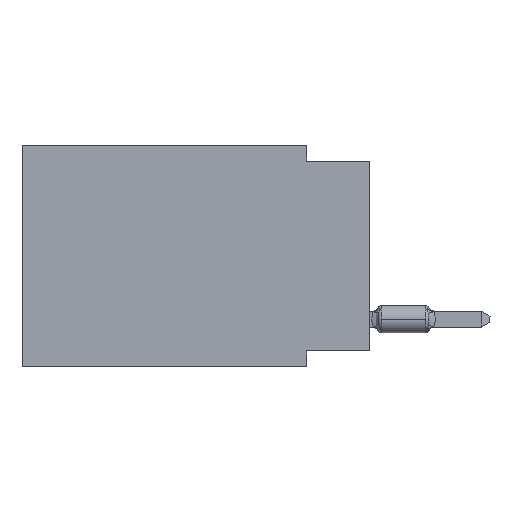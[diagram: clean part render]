
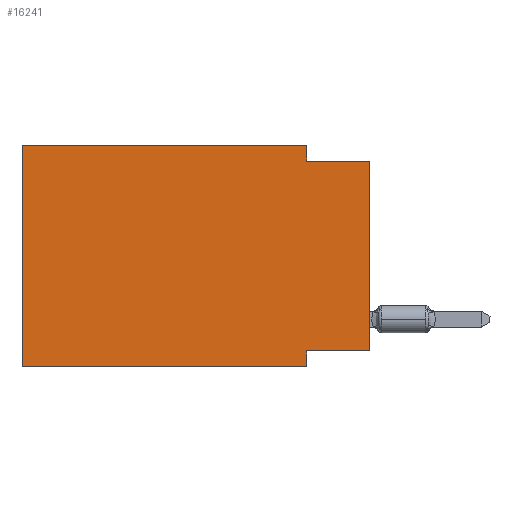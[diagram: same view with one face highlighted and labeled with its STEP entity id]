
A CAD part, left-side view. The second image highlights one B-rep face of the part: STEP entity #16241.
In plain terms, the highlighted planar face has unit normal (-1, 0, 0).
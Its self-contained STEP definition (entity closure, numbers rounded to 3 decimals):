
#185 = CARTESIAN_POINT ( 'NONE',  ( 0., 2.54, 0. ) ) ;
#246 = DIRECTION ( 'NONE',  ( 1., 0., 0. ) ) ;
#459 = CARTESIAN_POINT ( 'NONE',  ( 0., 0., -8.255 ) ) ;
#658 = LINE ( 'NONE', #14765, #14138 ) ;
#840 = VERTEX_POINT ( 'NONE', #3862 ) ;
#853 = VECTOR ( 'NONE', #5215, 1000. ) ;
#1459 = LINE ( 'NONE', #459, #10070 ) ;
#1527 = ORIENTED_EDGE ( 'NONE', *, *, #9915, .F. ) ;
#1926 = LINE ( 'NONE', #8041, #5080 ) ;
#2271 = LINE ( 'NONE', #2593, #2437 ) ;
#2437 = VECTOR ( 'NONE', #10041, 1000. ) ;
#2534 = EDGE_CURVE ( 'NONE', #9125, #10324, #11504, .T. ) ;
#2593 = CARTESIAN_POINT ( 'NONE',  ( 0., 2.54, -8.89 ) ) ;
#2864 = VERTEX_POINT ( 'NONE', #6585 ) ;
#2970 = ORIENTED_EDGE ( 'NONE', *, *, #7708, .F. ) ;
#3040 = VERTEX_POINT ( 'NONE', #4750 ) ;
#3373 = DIRECTION ( 'NONE',  ( 0., -1., 0. ) ) ;
#3577 = ORIENTED_EDGE ( 'NONE', *, *, #12218, .F. ) ;
#3752 = VECTOR ( 'NONE', #6814, 1000. ) ;
#3862 = CARTESIAN_POINT ( 'NONE',  ( 0., 13.97, -8.89 ) ) ;
#3876 = EDGE_LOOP ( 'NONE', ( #8422, #14463, #13564, #1527, #2970, #4227, #12075, #3577 ) ) ;
#4227 = ORIENTED_EDGE ( 'NONE', *, *, #6382, .T. ) ;
#4547 = CARTESIAN_POINT ( 'NONE',  ( 0., 2.54, -0.635 ) ) ;
#4742 = CARTESIAN_POINT ( 'NONE',  ( 0., 13.97, 0. ) ) ;
#4750 = CARTESIAN_POINT ( 'NONE',  ( 0., 2.54, -8.89 ) ) ;
#5080 = VECTOR ( 'NONE', #10938, 1000. ) ;
#5215 = DIRECTION ( 'NONE',  ( 0., 0., -1. ) ) ;
#5586 = VECTOR ( 'NONE', #8556, 1000. ) ;
#5631 = EDGE_CURVE ( 'NONE', #10324, #10305, #658, .T. ) ;
#6362 = DIRECTION ( 'NONE',  ( 0., 0., -1. ) ) ;
#6382 = EDGE_CURVE ( 'NONE', #840, #3040, #8968, .T. ) ;
#6585 = CARTESIAN_POINT ( 'NONE',  ( 0., 13.97, 0. ) ) ;
#6814 = DIRECTION ( 'NONE',  ( 0., 0., 1. ) ) ;
#7611 = VERTEX_POINT ( 'NONE', #14409 ) ;
#7708 = EDGE_CURVE ( 'NONE', #840, #2864, #16056, .T. ) ;
#8041 = CARTESIAN_POINT ( 'NONE',  ( 0., 13.97, 0. ) ) ;
#8422 = ORIENTED_EDGE ( 'NONE', *, *, #12714, .T. ) ;
#8556 = DIRECTION ( 'NONE',  ( 0., 0., 1. ) ) ;
#8935 = PLANE ( 'NONE',  #9315 ) ;
#8968 = LINE ( 'NONE', #15800, #10439 ) ;
#9125 = VERTEX_POINT ( 'NONE', #13109 ) ;
#9308 = LINE ( 'NONE', #10715, #3752 ) ;
#9315 = AXIS2_PLACEMENT_3D ( 'NONE', #12565, #246, #6362 ) ;
#9582 = VERTEX_POINT ( 'NONE', #15802 ) ;
#9612 = EDGE_CURVE ( 'NONE', #7611, #3040, #2271, .T. ) ;
#9915 = EDGE_CURVE ( 'NONE', #2864, #9125, #1926, .T. ) ;
#10041 = DIRECTION ( 'NONE',  ( 0., 0., -1. ) ) ;
#10070 = VECTOR ( 'NONE', #11957, 1000. ) ;
#10305 = VERTEX_POINT ( 'NONE', #15850 ) ;
#10324 = VERTEX_POINT ( 'NONE', #4547 ) ;
#10439 = VECTOR ( 'NONE', #10864, 1000. ) ;
#10715 = CARTESIAN_POINT ( 'NONE',  ( 0., 0., 0. ) ) ;
#10864 = DIRECTION ( 'NONE',  ( 0., -1., 0. ) ) ;
#10938 = DIRECTION ( 'NONE',  ( 0., -1., 0. ) ) ;
#11504 = LINE ( 'NONE', #185, #853 ) ;
#11957 = DIRECTION ( 'NONE',  ( 0., 1., 0. ) ) ;
#12075 = ORIENTED_EDGE ( 'NONE', *, *, #9612, .F. ) ;
#12218 = EDGE_CURVE ( 'NONE', #9582, #7611, #1459, .T. ) ;
#12565 = CARTESIAN_POINT ( 'NONE',  ( 0., 13.97, 0. ) ) ;
#12714 = EDGE_CURVE ( 'NONE', #9582, #10305, #9308, .T. ) ;
#13109 = CARTESIAN_POINT ( 'NONE',  ( 0., 2.54, 0. ) ) ;
#13564 = ORIENTED_EDGE ( 'NONE', *, *, #2534, .F. ) ;
#13710 = FACE_OUTER_BOUND ( 'NONE', #3876, .T. ) ;
#14138 = VECTOR ( 'NONE', #3373, 1000. ) ;
#14409 = CARTESIAN_POINT ( 'NONE',  ( 0., 2.54, -8.255 ) ) ;
#14463 = ORIENTED_EDGE ( 'NONE', *, *, #5631, .F. ) ;
#14765 = CARTESIAN_POINT ( 'NONE',  ( 0., 0., -0.635 ) ) ;
#15800 = CARTESIAN_POINT ( 'NONE',  ( 0., 13.97, -8.89 ) ) ;
#15802 = CARTESIAN_POINT ( 'NONE',  ( 0., 0., -8.255 ) ) ;
#15850 = CARTESIAN_POINT ( 'NONE',  ( 0., 0., -0.635 ) ) ;
#16056 = LINE ( 'NONE', #4742, #5586 ) ;
#16241 = ADVANCED_FACE ( 'NONE', ( #13710 ), #8935, .F. ) ;
